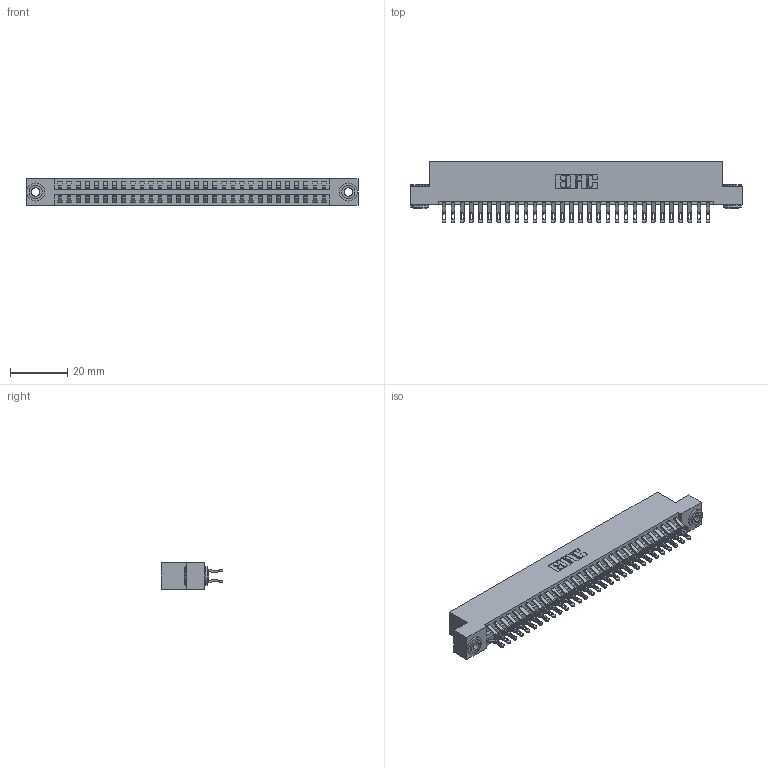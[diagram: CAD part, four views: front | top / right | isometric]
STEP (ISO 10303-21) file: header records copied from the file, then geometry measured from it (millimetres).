
FILE_DESCRIPTION (( 'STEP AP203' ), '1' );
FILE_NAME ('396-060-555-203.STEP', '2018-09-08T13:35:17', ( '' ), ( '' ), 'SwSTEP 2.0', 'SolidWorks 2016', '' );
FILE_SCHEMA (( 'CONFIG_CONTROL_DESIGN' ));
Length unit declared in the file: inch
Products named in the file (4): 346 Part_Flush Mounting Lugs - 0.156 Dia-TH; 345-292-001_555 Tail; 345-250-002_345-250-002-102; 396-060-555-203
Assembly tree (63 placements, depth 2):
  396-060-555-203
    346 Part_Flush Mounting Lugs - 0.156 Dia-TH
    345-292-001_555 Tail  x60
    345-250-002_345-250-002-102  x2
Bounding box: 115.82 x 21.46 x 9.4 mm (x, y, z)
Volume: 11394.5 mm3; surface area: 16308.4 mm2
Topology: 63 solids, 63 shells, 3640 faces, 11385 edges, 7586 vertices
Faces by surface type: plane 2066, cylinder 1566, cone 8
Entity records: 22170 total; most frequent: CARTESIAN_POINT 3681, ORIENTED_EDGE 3578, DIRECTION 3295, EDGE_CURVE 1789, VECTOR 1493, LINE 1493, VERTEX_POINT 1190, AXIS2_PLACEMENT_3D 901
